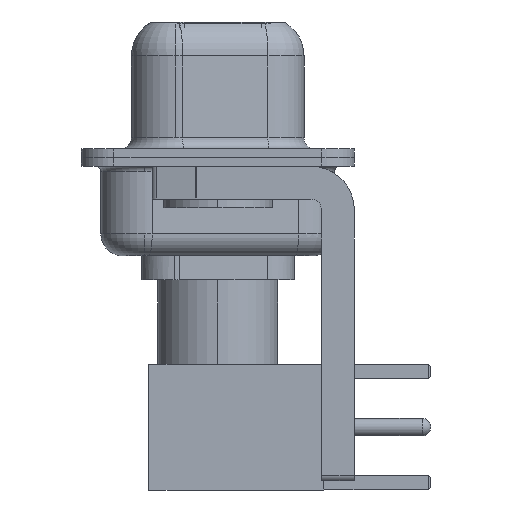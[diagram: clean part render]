
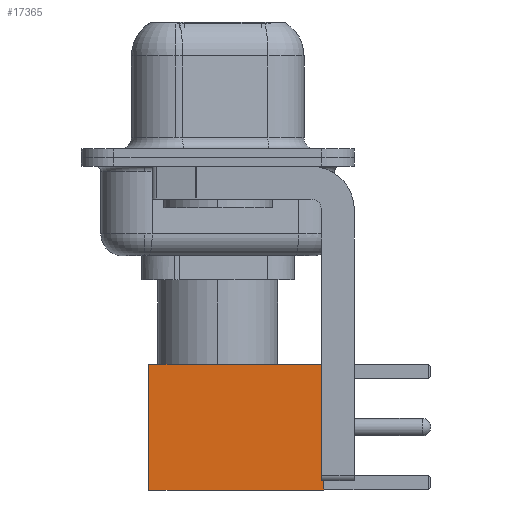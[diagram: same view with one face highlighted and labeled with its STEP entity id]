
A CAD part, left-side view. The second image highlights one B-rep face of the part: STEP entity #17365.
In plain terms, the highlighted face is planar.
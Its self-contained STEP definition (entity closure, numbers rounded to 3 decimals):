
#3 = VECTOR ( 'NONE', #16855, 1000. ) ;
#183 = EDGE_LOOP ( 'NONE', ( #15811, #18624, #17994, #10873 ) ) ;
#656 = VECTOR ( 'NONE', #4087, 1000. ) ;
#1466 = DIRECTION ( 'NONE',  ( 0., 1., 0. ) ) ;
#1992 = VERTEX_POINT ( 'NONE', #8979 ) ;
#2316 = LINE ( 'NONE', #9660, #3 ) ;
#2887 = EDGE_CURVE ( 'NONE', #10662, #1992, #12875, .T. ) ;
#3007 = PLANE ( 'NONE',  #3574 ) ;
#3127 = VECTOR ( 'NONE', #8063, 1000. ) ;
#3268 = VECTOR ( 'NONE', #7944, 1000. ) ;
#3574 = AXIS2_PLACEMENT_3D ( 'NONE', #12804, #1466, #6827 ) ;
#4087 = DIRECTION ( 'NONE',  ( 0., 0., -1. ) ) ;
#4359 = CARTESIAN_POINT ( 'NONE',  ( 2.875, 2.875, 0. ) ) ;
#5623 = CARTESIAN_POINT ( 'NONE',  ( -2.875, 2.875, 8. ) ) ;
#5919 = EDGE_CURVE ( 'NONE', #11723, #1992, #9200, .T. ) ;
#6620 = VERTEX_POINT ( 'NONE', #17586 ) ;
#6827 = DIRECTION ( 'NONE',  ( 0., 0., 1. ) ) ;
#7104 = EDGE_CURVE ( 'NONE', #6620, #11723, #15432, .T. ) ;
#7944 = DIRECTION ( 'NONE',  ( -1., 0., 0. ) ) ;
#8063 = DIRECTION ( 'NONE',  ( 0., 0., -1. ) ) ;
#8647 = EDGE_CURVE ( 'NONE', #6620, #10662, #2316, .T. ) ;
#8979 = CARTESIAN_POINT ( 'NONE',  ( -2.875, 2.875, 0. ) ) ;
#9200 = LINE ( 'NONE', #9390, #3268 ) ;
#9390 = CARTESIAN_POINT ( 'NONE',  ( 0., 2.875, 0. ) ) ;
#9660 = CARTESIAN_POINT ( 'NONE',  ( 0., 2.875, 8. ) ) ;
#10662 = VERTEX_POINT ( 'NONE', #5623 ) ;
#10873 = ORIENTED_EDGE ( 'NONE', *, *, #8647, .F. ) ;
#11723 = VERTEX_POINT ( 'NONE', #4359 ) ;
#12498 = CARTESIAN_POINT ( 'NONE',  ( 2.875, 2.875, 0. ) ) ;
#12719 = FACE_OUTER_BOUND ( 'NONE', #183, .T. ) ;
#12804 = CARTESIAN_POINT ( 'NONE',  ( 2.875, 2.875, 0. ) ) ;
#12875 = LINE ( 'NONE', #17383, #656 ) ;
#15432 = LINE ( 'NONE', #12498, #3127 ) ;
#15811 = ORIENTED_EDGE ( 'NONE', *, *, #7104, .T. ) ;
#16855 = DIRECTION ( 'NONE',  ( -1., 0., 0. ) ) ;
#17365 = ADVANCED_FACE ( 'NONE', ( #12719 ), #3007, .T. ) ;
#17383 = CARTESIAN_POINT ( 'NONE',  ( -2.875, 2.875, 0. ) ) ;
#17586 = CARTESIAN_POINT ( 'NONE',  ( 2.875, 2.875, 8. ) ) ;
#17994 = ORIENTED_EDGE ( 'NONE', *, *, #2887, .F. ) ;
#18624 = ORIENTED_EDGE ( 'NONE', *, *, #5919, .T. ) ;
